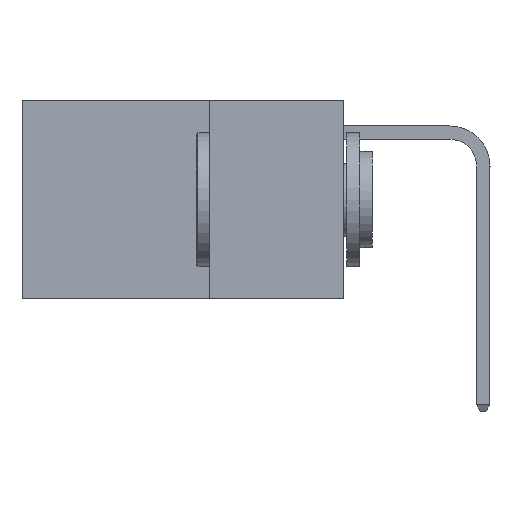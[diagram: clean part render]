
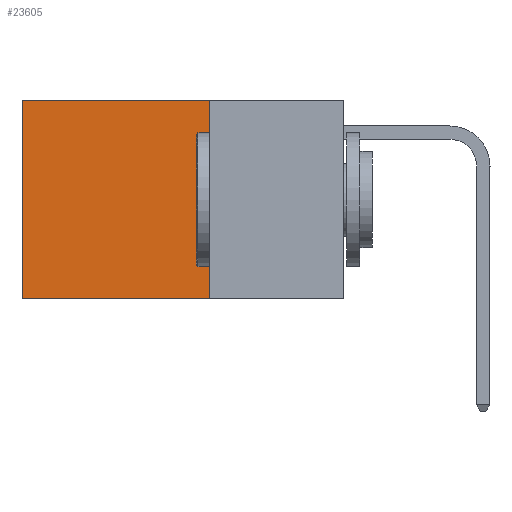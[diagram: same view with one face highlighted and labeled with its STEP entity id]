
A CAD part, left-side view. The second image highlights one B-rep face of the part: STEP entity #23605.
In plain terms, the highlighted planar face has unit normal (-1, 0, 0).
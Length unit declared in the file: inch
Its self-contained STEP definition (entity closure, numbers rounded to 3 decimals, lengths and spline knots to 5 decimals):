
#57 = CARTESIAN_POINT ( 'NONE',  ( 0.2625, 0.6, 0. ) ) ;
#750 = DIRECTION ( 'NONE',  ( 0., 0., -1. ) ) ;
#2072 = VERTEX_POINT ( 'NONE', #12346 ) ;
#2469 = VERTEX_POINT ( 'NONE', #57 ) ;
#2861 = VECTOR ( 'NONE', #29852, 39.37008 ) ;
#3806 = LINE ( 'NONE', #7881, #21070 ) ;
#4360 = LINE ( 'NONE', #27557, #2861 ) ;
#5071 = ORIENTED_EDGE ( 'NONE', *, *, #16975, .T. ) ;
#7078 = VECTOR ( 'NONE', #17852, 39.37008 ) ;
#7881 = CARTESIAN_POINT ( 'NONE',  ( 0.2625, 0.25, 0. ) ) ;
#8225 = ORIENTED_EDGE ( 'NONE', *, *, #15592, .F. ) ;
#8595 = EDGE_LOOP ( 'NONE', ( #19786, #15868, #8225, #5071 ) ) ;
#10833 = VERTEX_POINT ( 'NONE', #28339 ) ;
#12346 = CARTESIAN_POINT ( 'NONE',  ( 0.2625, 0.25, 0. ) ) ;
#12582 = LINE ( 'NONE', #13135, #7078 ) ;
#13135 = CARTESIAN_POINT ( 'NONE',  ( 0.2625, 0.25, 0. ) ) ;
#14738 = AXIS2_PLACEMENT_3D ( 'NONE', #28679, #14880, #750 ) ;
#14880 = DIRECTION ( 'NONE',  ( 1., 0., 0. ) ) ;
#15592 = EDGE_CURVE ( 'NONE', #2072, #10833, #3806, .T. ) ;
#15868 = ORIENTED_EDGE ( 'NONE', *, *, #22606, .F. ) ;
#16975 = EDGE_CURVE ( 'NONE', #2072, #2469, #12582, .T. ) ;
#17210 = DIRECTION ( 'NONE',  ( 0., 0., -1. ) ) ;
#17852 = DIRECTION ( 'NONE',  ( 0., 1., 0. ) ) ;
#19786 = ORIENTED_EDGE ( 'NONE', *, *, #24135, .T. ) ;
#20072 = VECTOR ( 'NONE', #24473, 39.37008 ) ;
#21070 = VECTOR ( 'NONE', #17210, 39.37008 ) ;
#21792 = PLANE ( 'NONE',  #14738 ) ;
#22606 = EDGE_CURVE ( 'NONE', #10833, #26186, #4360, .T. ) ;
#22623 = CARTESIAN_POINT ( 'NONE',  ( 0.2625, 0.6, -0.37 ) ) ;
#23316 = FACE_OUTER_BOUND ( 'NONE', #8595, .T. ) ;
#23605 = ADVANCED_FACE ( 'NONE', ( #23316 ), #21792, .F. ) ;
#24135 = EDGE_CURVE ( 'NONE', #2469, #26186, #26183, .T. ) ;
#24473 = DIRECTION ( 'NONE',  ( 0., 0., -1. ) ) ;
#26183 = LINE ( 'NONE', #26767, #20072 ) ;
#26186 = VERTEX_POINT ( 'NONE', #22623 ) ;
#26767 = CARTESIAN_POINT ( 'NONE',  ( 0.2625, 0.6, 0. ) ) ;
#27557 = CARTESIAN_POINT ( 'NONE',  ( 0.2625, 0.25, -0.37 ) ) ;
#28339 = CARTESIAN_POINT ( 'NONE',  ( 0.2625, 0.25, -0.37 ) ) ;
#28679 = CARTESIAN_POINT ( 'NONE',  ( 0.2625, 0.25, 0. ) ) ;
#29852 = DIRECTION ( 'NONE',  ( 0., 1., 0. ) ) ;
